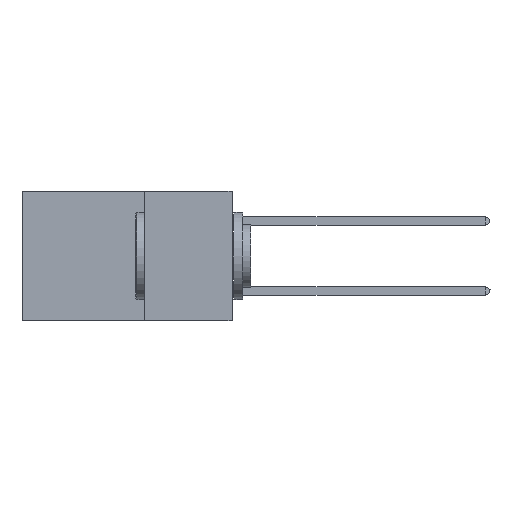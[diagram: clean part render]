
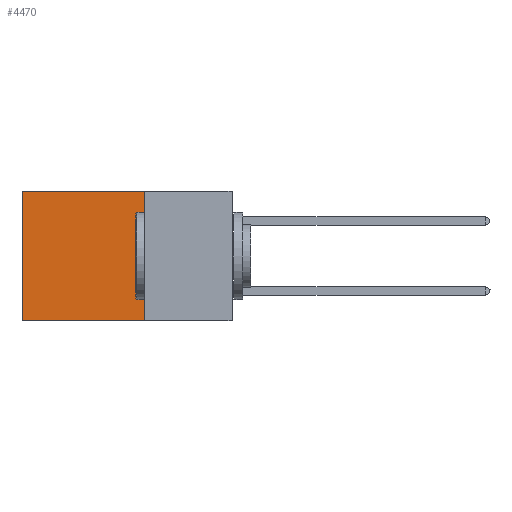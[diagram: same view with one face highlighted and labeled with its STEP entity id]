
A CAD part, left-side view. The second image highlights one B-rep face of the part: STEP entity #4470.
In plain terms, the highlighted planar face has unit normal (-1, 0, 0).
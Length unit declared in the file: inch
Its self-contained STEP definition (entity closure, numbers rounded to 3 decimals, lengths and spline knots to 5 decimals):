
#285 = VERTEX_POINT ( 'NONE', #4515 ) ;
#996 = FACE_OUTER_BOUND ( 'NONE', #21353, .T. ) ;
#1475 = CARTESIAN_POINT ( 'NONE',  ( 0.2875, 0.6, -0.37 ) ) ;
#1936 = CARTESIAN_POINT ( 'NONE',  ( 0.2875, 0.25, -0.37 ) ) ;
#3155 = PLANE ( 'NONE',  #6709 ) ;
#3484 = CARTESIAN_POINT ( 'NONE',  ( 0.2875, 0.6, 0. ) ) ;
#4113 = LINE ( 'NONE', #12764, #20471 ) ;
#4265 = LINE ( 'NONE', #3484, #12897 ) ;
#4470 = ADVANCED_FACE ( 'NONE', ( #996 ), #3155, .F. ) ;
#4515 = CARTESIAN_POINT ( 'NONE',  ( 0.2875, 0.25, 0. ) ) ;
#5902 = ORIENTED_EDGE ( 'NONE', *, *, #20100, .T. ) ;
#6709 = AXIS2_PLACEMENT_3D ( 'NONE', #32177, #30254, #30905 ) ;
#7542 = VECTOR ( 'NONE', #15235, 39.37008 ) ;
#8987 = CARTESIAN_POINT ( 'NONE',  ( 0.2875, 0.6, 0. ) ) ;
#10937 = EDGE_CURVE ( 'NONE', #29397, #12509, #17782, .T. ) ;
#12497 = DIRECTION ( 'NONE',  ( 0., 1., 0. ) ) ;
#12509 = VERTEX_POINT ( 'NONE', #1475 ) ;
#12764 = CARTESIAN_POINT ( 'NONE',  ( 0.2875, 0.25, 0. ) ) ;
#12897 = VECTOR ( 'NONE', #29471, 39.37008 ) ;
#15235 = DIRECTION ( 'NONE',  ( 0., 0., -1. ) ) ;
#16925 = ORIENTED_EDGE ( 'NONE', *, *, #35211, .T. ) ;
#17782 = LINE ( 'NONE', #34637, #25080 ) ;
#20100 = EDGE_CURVE ( 'NONE', #285, #25863, #4113, .T. ) ;
#20471 = VECTOR ( 'NONE', #12497, 39.37008 ) ;
#21353 = EDGE_LOOP ( 'NONE', ( #16925, #36477, #30369, #5902 ) ) ;
#25080 = VECTOR ( 'NONE', #37544, 39.37008 ) ;
#25863 = VERTEX_POINT ( 'NONE', #8987 ) ;
#26184 = EDGE_CURVE ( 'NONE', #285, #29397, #30649, .T. ) ;
#29397 = VERTEX_POINT ( 'NONE', #1936 ) ;
#29471 = DIRECTION ( 'NONE',  ( 0., 0., -1. ) ) ;
#30254 = DIRECTION ( 'NONE',  ( 1., 0., 0. ) ) ;
#30369 = ORIENTED_EDGE ( 'NONE', *, *, #26184, .F. ) ;
#30649 = LINE ( 'NONE', #35237, #7542 ) ;
#30905 = DIRECTION ( 'NONE',  ( 0., 0., -1. ) ) ;
#32177 = CARTESIAN_POINT ( 'NONE',  ( 0.2875, 0.25, 0. ) ) ;
#34637 = CARTESIAN_POINT ( 'NONE',  ( 0.2875, 0.25, -0.37 ) ) ;
#35211 = EDGE_CURVE ( 'NONE', #25863, #12509, #4265, .T. ) ;
#35237 = CARTESIAN_POINT ( 'NONE',  ( 0.2875, 0.25, 0. ) ) ;
#36477 = ORIENTED_EDGE ( 'NONE', *, *, #10937, .F. ) ;
#37544 = DIRECTION ( 'NONE',  ( 0., 1., 0. ) ) ;
